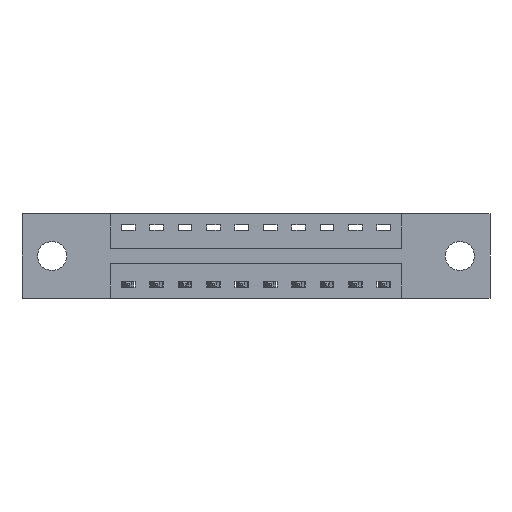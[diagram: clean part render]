
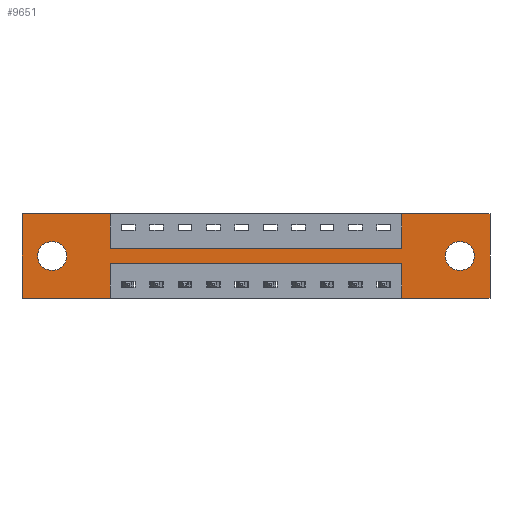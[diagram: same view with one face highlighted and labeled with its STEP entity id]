
A CAD part, front view. The second image highlights one B-rep face of the part: STEP entity #9651.
In plain terms, the highlighted planar face has unit normal (0, -1, 0).
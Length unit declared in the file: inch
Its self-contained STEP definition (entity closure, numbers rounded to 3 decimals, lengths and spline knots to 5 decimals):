
#62 = ORIENTED_EDGE ( 'NONE', *, *, #10196, .T. ) ;
#265 = VERTEX_POINT ( 'NONE', #4690 ) ;
#368 = LINE ( 'NONE', #9130, #2904 ) ;
#419 = CARTESIAN_POINT ( 'NONE',  ( 0.1325, 0., -0.121 ) ) ;
#465 = EDGE_CURVE ( 'NONE', #6385, #4271, #6219, .T. ) ;
#500 = LINE ( 'NONE', #4673, #9110 ) ;
#832 = VERTEX_POINT ( 'NONE', #7660 ) ;
#917 = ORIENTED_EDGE ( 'NONE', *, *, #4416, .F. ) ;
#1090 = CIRCLE ( 'NONE', #10499, 0.064 ) ;
#1243 = CARTESIAN_POINT ( 'NONE',  ( 2.06, 0., 0. ) ) ;
#1324 = LINE ( 'NONE', #9664, #4380 ) ;
#1423 = ORIENTED_EDGE ( 'NONE', *, *, #3361, .F. ) ;
#1462 = VECTOR ( 'NONE', #3255, 39.37008 ) ;
#1478 = DIRECTION ( 'NONE',  ( 1., 0., 0. ) ) ;
#1495 = DIRECTION ( 'NONE',  ( 0., 1., 0. ) ) ;
#1499 = VERTEX_POINT ( 'NONE', #5061 ) ;
#1538 = VECTOR ( 'NONE', #8902, 39.37008 ) ;
#1706 = CARTESIAN_POINT ( 'NONE',  ( 2.06, 0., -0.37 ) ) ;
#1774 = EDGE_CURVE ( 'NONE', #7189, #265, #1324, .T. ) ;
#1791 = VERTEX_POINT ( 'NONE', #3239 ) ;
#2008 = ORIENTED_EDGE ( 'NONE', *, *, #10511, .F. ) ;
#2025 = DIRECTION ( 'NONE',  ( 0., 0., 1. ) ) ;
#2050 = ORIENTED_EDGE ( 'NONE', *, *, #1774, .F. ) ;
#2152 = CARTESIAN_POINT ( 'NONE',  ( 0., 0., -0.37 ) ) ;
#2322 = DIRECTION ( 'NONE',  ( 0., 0., -1. ) ) ;
#2342 = AXIS2_PLACEMENT_3D ( 'NONE', #4739, #3573, #3279 ) ;
#2380 = DIRECTION ( 'NONE',  ( 0., 1., 0. ) ) ;
#2390 = FACE_BOUND ( 'NONE', #4453, .T. ) ;
#2477 = CARTESIAN_POINT ( 'NONE',  ( 1.9275, 0., -0.185 ) ) ;
#2512 = ORIENTED_EDGE ( 'NONE', *, *, #5631, .F. ) ;
#2666 = FACE_BOUND ( 'NONE', #5801, .T. ) ;
#2712 = CARTESIAN_POINT ( 'NONE',  ( 1.6725, 0., -0.37 ) ) ;
#2739 = EDGE_LOOP ( 'NONE', ( #2008, #6633, #2050, #917, #2512, #1423, #7849, #7491, #6210, #7103, #9872, #8824 ) ) ;
#2795 = VECTOR ( 'NONE', #5449, 39.37008 ) ;
#2904 = VECTOR ( 'NONE', #5489, 39.37008 ) ;
#3056 = VECTOR ( 'NONE', #3360, 39.37008 ) ;
#3239 = CARTESIAN_POINT ( 'NONE',  ( 0., 0., 0. ) ) ;
#3255 = DIRECTION ( 'NONE',  ( 1., 0., 0. ) ) ;
#3279 = DIRECTION ( 'NONE',  ( 0., 0., -1. ) ) ;
#3360 = DIRECTION ( 'NONE',  ( -1., 0., 0. ) ) ;
#3361 = EDGE_CURVE ( 'NONE', #10019, #4101, #6090, .T. ) ;
#3368 = CARTESIAN_POINT ( 'NONE',  ( 1.9275, 0., -0.185 ) ) ;
#3514 = VERTEX_POINT ( 'NONE', #419 ) ;
#3526 = VECTOR ( 'NONE', #5312, 39.37008 ) ;
#3538 = PLANE ( 'NONE',  #2342 ) ;
#3573 = DIRECTION ( 'NONE',  ( 0., -1., 0. ) ) ;
#3960 = EDGE_CURVE ( 'NONE', #4271, #10019, #7265, .T. ) ;
#3979 = CARTESIAN_POINT ( 'NONE',  ( 0.1325, 0., -0.185 ) ) ;
#4101 = VERTEX_POINT ( 'NONE', #1243 ) ;
#4231 = VERTEX_POINT ( 'NONE', #6027 ) ;
#4271 = VERTEX_POINT ( 'NONE', #4279 ) ;
#4279 = CARTESIAN_POINT ( 'NONE',  ( 1.6725, 0., -0.15 ) ) ;
#4380 = VECTOR ( 'NONE', #7162, 39.37008 ) ;
#4416 = EDGE_CURVE ( 'NONE', #8877, #7189, #8220, .T. ) ;
#4453 = EDGE_LOOP ( 'NONE', ( #7666, #8118 ) ) ;
#4673 = CARTESIAN_POINT ( 'NONE',  ( 0., 0., 0. ) ) ;
#4690 = CARTESIAN_POINT ( 'NONE',  ( 1.6725, 0., -0.22 ) ) ;
#4739 = CARTESIAN_POINT ( 'NONE',  ( 0., 0., -0.37 ) ) ;
#4768 = CARTESIAN_POINT ( 'NONE',  ( 2.06, 0., 0. ) ) ;
#4854 = CARTESIAN_POINT ( 'NONE',  ( 0., 0., 0. ) ) ;
#5061 = CARTESIAN_POINT ( 'NONE',  ( 0.3875, 0., 0. ) ) ;
#5115 = DIRECTION ( 'NONE',  ( 0., 0., -1. ) ) ;
#5237 = EDGE_CURVE ( 'NONE', #265, #832, #8669, .T. ) ;
#5288 = CARTESIAN_POINT ( 'NONE',  ( 0.1325, 0., -0.249 ) ) ;
#5312 = DIRECTION ( 'NONE',  ( -1., 0., 0. ) ) ;
#5314 = CARTESIAN_POINT ( 'NONE',  ( 1.9275, 0., -0.121 ) ) ;
#5449 = DIRECTION ( 'NONE',  ( 0., 0., -1. ) ) ;
#5489 = DIRECTION ( 'NONE',  ( 0., 0., 1. ) ) ;
#5631 = EDGE_CURVE ( 'NONE', #4101, #8877, #9357, .T. ) ;
#5801 = EDGE_LOOP ( 'NONE', ( #62, #7346 ) ) ;
#5862 = VERTEX_POINT ( 'NONE', #5288 ) ;
#5977 = CARTESIAN_POINT ( 'NONE',  ( 0.3875, 0., 0. ) ) ;
#6010 = CIRCLE ( 'NONE', #9839, 0.064 ) ;
#6027 = CARTESIAN_POINT ( 'NONE',  ( 0., 0., -0.37 ) ) ;
#6090 = LINE ( 'NONE', #4854, #1462 ) ;
#6167 = LINE ( 'NONE', #8991, #1538 ) ;
#6210 = ORIENTED_EDGE ( 'NONE', *, *, #6814, .F. ) ;
#6211 = AXIS2_PLACEMENT_3D ( 'NONE', #2477, #2380, #2322 ) ;
#6219 = LINE ( 'NONE', #10421, #7008 ) ;
#6243 = VERTEX_POINT ( 'NONE', #8257 ) ;
#6385 = VERTEX_POINT ( 'NONE', #7573 ) ;
#6569 = VECTOR ( 'NONE', #8606, 39.37008 ) ;
#6595 = AXIS2_PLACEMENT_3D ( 'NONE', #3368, #1495, #5115 ) ;
#6633 = ORIENTED_EDGE ( 'NONE', *, *, #5237, .F. ) ;
#6669 = LINE ( 'NONE', #5977, #10422 ) ;
#6691 = EDGE_CURVE ( 'NONE', #9008, #9203, #9909, .T. ) ;
#6814 = EDGE_CURVE ( 'NONE', #1499, #6385, #6669, .T. ) ;
#6969 = FACE_OUTER_BOUND ( 'NONE', #2739, .T. ) ;
#7008 = VECTOR ( 'NONE', #1478, 39.37008 ) ;
#7103 = ORIENTED_EDGE ( 'NONE', *, *, #7725, .F. ) ;
#7162 = DIRECTION ( 'NONE',  ( 0., 0., 1. ) ) ;
#7189 = VERTEX_POINT ( 'NONE', #2712 ) ;
#7265 = LINE ( 'NONE', #7750, #8815 ) ;
#7292 = EDGE_CURVE ( 'NONE', #6243, #4231, #8883, .T. ) ;
#7346 = ORIENTED_EDGE ( 'NONE', *, *, #6691, .T. ) ;
#7411 = CARTESIAN_POINT ( 'NONE',  ( 1.9275, 0., -0.249 ) ) ;
#7416 = EDGE_CURVE ( 'NONE', #3514, #5862, #6010, .T. ) ;
#7491 = ORIENTED_EDGE ( 'NONE', *, *, #465, .F. ) ;
#7528 = EDGE_CURVE ( 'NONE', #4231, #1791, #368, .T. ) ;
#7573 = CARTESIAN_POINT ( 'NONE',  ( 0.3875, 0., -0.15 ) ) ;
#7660 = CARTESIAN_POINT ( 'NONE',  ( 0.3875, 0., -0.22 ) ) ;
#7666 = ORIENTED_EDGE ( 'NONE', *, *, #7416, .T. ) ;
#7693 = DIRECTION ( 'NONE',  ( 0., 0., 1. ) ) ;
#7725 = EDGE_CURVE ( 'NONE', #1791, #1499, #500, .T. ) ;
#7750 = CARTESIAN_POINT ( 'NONE',  ( 1.6725, 0., 0. ) ) ;
#7849 = ORIENTED_EDGE ( 'NONE', *, *, #3960, .F. ) ;
#8118 = ORIENTED_EDGE ( 'NONE', *, *, #8840, .T. ) ;
#8220 = LINE ( 'NONE', #10079, #3526 ) ;
#8257 = CARTESIAN_POINT ( 'NONE',  ( 0.3875, 0., -0.37 ) ) ;
#8303 = DIRECTION ( 'NONE',  ( 0., 0., -1. ) ) ;
#8375 = DIRECTION ( 'NONE',  ( 1., 0., 0. ) ) ;
#8437 = DIRECTION ( 'NONE',  ( 0., 0., 1. ) ) ;
#8606 = DIRECTION ( 'NONE',  ( -1., 0., 0. ) ) ;
#8669 = LINE ( 'NONE', #9746, #6569 ) ;
#8771 = CARTESIAN_POINT ( 'NONE',  ( 1.6725, 0., 0. ) ) ;
#8815 = VECTOR ( 'NONE', #2025, 39.37008 ) ;
#8824 = ORIENTED_EDGE ( 'NONE', *, *, #7292, .F. ) ;
#8840 = EDGE_CURVE ( 'NONE', #5862, #3514, #1090, .T. ) ;
#8877 = VERTEX_POINT ( 'NONE', #1706 ) ;
#8883 = LINE ( 'NONE', #2152, #3056 ) ;
#8902 = DIRECTION ( 'NONE',  ( 0., 0., -1. ) ) ;
#8991 = CARTESIAN_POINT ( 'NONE',  ( 0.3875, 0., -0.37 ) ) ;
#9008 = VERTEX_POINT ( 'NONE', #7411 ) ;
#9110 = VECTOR ( 'NONE', #8375, 39.37008 ) ;
#9130 = CARTESIAN_POINT ( 'NONE',  ( 0., 0., 0. ) ) ;
#9203 = VERTEX_POINT ( 'NONE', #5314 ) ;
#9324 = CARTESIAN_POINT ( 'NONE',  ( 0.1325, 0., -0.185 ) ) ;
#9332 = DIRECTION ( 'NONE',  ( 0., 1., 0. ) ) ;
#9357 = LINE ( 'NONE', #4768, #2795 ) ;
#9598 = CIRCLE ( 'NONE', #6211, 0.064 ) ;
#9651 = ADVANCED_FACE ( 'NONE', ( #2666, #2390, #6969 ), #3538, .T. ) ;
#9664 = CARTESIAN_POINT ( 'NONE',  ( 1.6725, 0., -0.37 ) ) ;
#9746 = CARTESIAN_POINT ( 'NONE',  ( 0.3875, 0., -0.22 ) ) ;
#9839 = AXIS2_PLACEMENT_3D ( 'NONE', #3979, #10393, #7693 ) ;
#9872 = ORIENTED_EDGE ( 'NONE', *, *, #7528, .F. ) ;
#9909 = CIRCLE ( 'NONE', #6595, 0.064 ) ;
#10019 = VERTEX_POINT ( 'NONE', #8771 ) ;
#10079 = CARTESIAN_POINT ( 'NONE',  ( 0., 0., -0.37 ) ) ;
#10196 = EDGE_CURVE ( 'NONE', #9203, #9008, #9598, .T. ) ;
#10393 = DIRECTION ( 'NONE',  ( 0., 1., 0. ) ) ;
#10421 = CARTESIAN_POINT ( 'NONE',  ( 0.3875, 0., -0.15 ) ) ;
#10422 = VECTOR ( 'NONE', #8303, 39.37008 ) ;
#10499 = AXIS2_PLACEMENT_3D ( 'NONE', #9324, #9332, #8437 ) ;
#10511 = EDGE_CURVE ( 'NONE', #832, #6243, #6167, .T. ) ;
